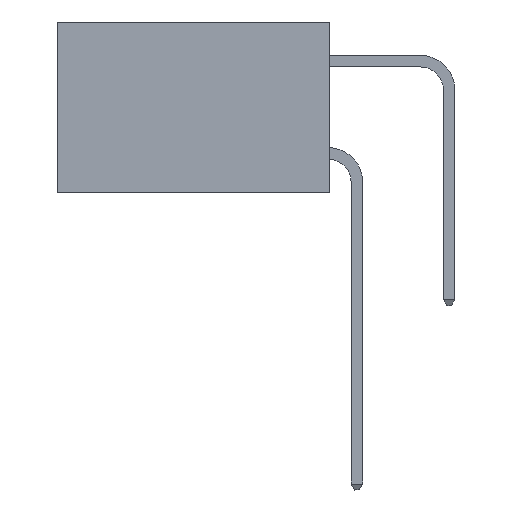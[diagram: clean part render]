
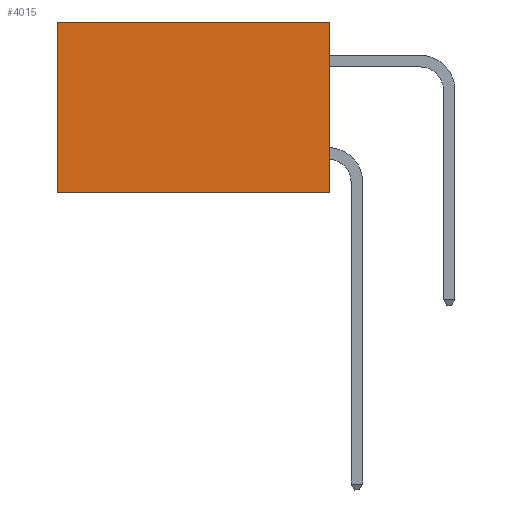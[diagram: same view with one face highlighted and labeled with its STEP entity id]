
A CAD part, left-side view. The second image highlights one B-rep face of the part: STEP entity #4015.
In plain terms, the highlighted planar face has unit normal (-1, 0, 0).
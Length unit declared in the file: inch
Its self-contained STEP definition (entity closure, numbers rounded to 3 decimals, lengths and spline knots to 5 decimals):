
#167 = ORIENTED_EDGE ( 'NONE', *, *, #5099, .F. ) ;
#2469 = DIRECTION ( 'NONE',  ( 1., 0., 0. ) ) ;
#2569 = DIRECTION ( 'NONE',  ( 0., 0., -1. ) ) ;
#4015 = ADVANCED_FACE ( 'NONE', ( #10434 ), #5974, .F. ) ;
#4838 = CARTESIAN_POINT ( 'NONE',  ( 0.277, 0., -0.37 ) ) ;
#5060 = EDGE_CURVE ( 'NONE', #20984, #17099, #9630, .T. ) ;
#5099 = EDGE_CURVE ( 'NONE', #18199, #20984, #20213, .T. ) ;
#5728 = CARTESIAN_POINT ( 'NONE',  ( 0.277, 0.59, 0. ) ) ;
#5974 = PLANE ( 'NONE',  #27061 ) ;
#6136 = LINE ( 'NONE', #14694, #22853 ) ;
#8808 = DIRECTION ( 'NONE',  ( 0., 0., -1. ) ) ;
#8878 = CARTESIAN_POINT ( 'NONE',  ( 0.277, 0., -0.37 ) ) ;
#8927 = VECTOR ( 'NONE', #9713, 39.37008 ) ;
#9329 = EDGE_LOOP ( 'NONE', ( #23060, #15173, #167, #28585 ) ) ;
#9630 = LINE ( 'NONE', #9754, #8927 ) ;
#9713 = DIRECTION ( 'NONE',  ( 0., 1., 0. ) ) ;
#9754 = CARTESIAN_POINT ( 'NONE',  ( 0.277, 0., -0.37 ) ) ;
#10434 = FACE_OUTER_BOUND ( 'NONE', #9329, .T. ) ;
#14694 = CARTESIAN_POINT ( 'NONE',  ( 0.277, 0., 0. ) ) ;
#15173 = ORIENTED_EDGE ( 'NONE', *, *, #5060, .F. ) ;
#16941 = DIRECTION ( 'NONE',  ( 0., 1., 0. ) ) ;
#16975 = DIRECTION ( 'NONE',  ( 0., 0., -1. ) ) ;
#17099 = VERTEX_POINT ( 'NONE', #26538 ) ;
#17728 = VERTEX_POINT ( 'NONE', #5728 ) ;
#18199 = VERTEX_POINT ( 'NONE', #27445 ) ;
#19100 = CARTESIAN_POINT ( 'NONE',  ( 0.277, 0.59, -0.37 ) ) ;
#19520 = VECTOR ( 'NONE', #8808, 39.37008 ) ;
#20167 = CARTESIAN_POINT ( 'NONE',  ( 0.277, 0., -0.37 ) ) ;
#20213 = LINE ( 'NONE', #8878, #19520 ) ;
#20984 = VERTEX_POINT ( 'NONE', #20167 ) ;
#21841 = VECTOR ( 'NONE', #16975, 39.37008 ) ;
#22853 = VECTOR ( 'NONE', #16941, 39.37008 ) ;
#23060 = ORIENTED_EDGE ( 'NONE', *, *, #27492, .T. ) ;
#26538 = CARTESIAN_POINT ( 'NONE',  ( 0.277, 0.59, -0.37 ) ) ;
#27010 = LINE ( 'NONE', #19100, #21841 ) ;
#27061 = AXIS2_PLACEMENT_3D ( 'NONE', #4838, #2469, #2569 ) ;
#27445 = CARTESIAN_POINT ( 'NONE',  ( 0.277, 0., 0. ) ) ;
#27492 = EDGE_CURVE ( 'NONE', #17728, #17099, #27010, .T. ) ;
#28220 = EDGE_CURVE ( 'NONE', #18199, #17728, #6136, .T. ) ;
#28585 = ORIENTED_EDGE ( 'NONE', *, *, #28220, .T. ) ;
